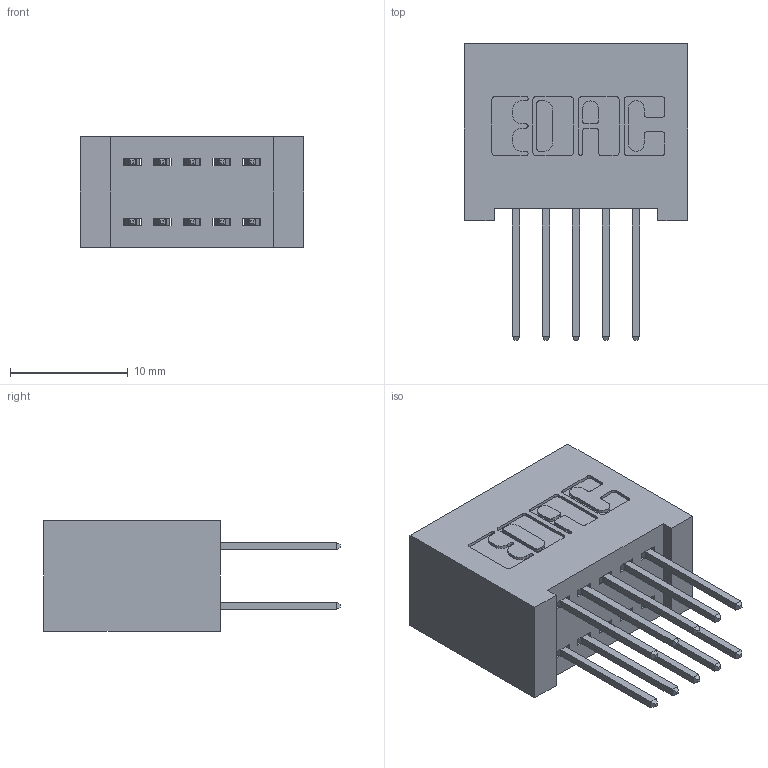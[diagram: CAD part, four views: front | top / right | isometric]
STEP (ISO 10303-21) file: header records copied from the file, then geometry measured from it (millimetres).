
FILE_DESCRIPTION (( 'STEP AP203' ), '1' );
FILE_NAME ('392-010-523-201.STEP', '2019-10-05T00:40:44', ( '' ), ( '' ), 'SwSTEP 2.0', 'SolidWorks 2016', '' );
FILE_SCHEMA (( 'CONFIG_CONTROL_DESIGN' ));
Length unit declared in the file: inch
Products named in the file (3): 392-010-523-201; 345-292-001_345-293-123; 342 Part_Lugless
Assembly tree (11 placements, depth 2):
  392-010-523-201
    342 Part_Lugless
    345-292-001_345-293-123  x10
Bounding box: 18.95 x 25.15 x 9.4 mm (x, y, z)
Volume: 1987.4 mm3; surface area: 2856.7 mm2
Topology: 11 solids, 11 shells, 622 faces, 1825 edges, 1202 vertices
Faces by surface type: plane 422, cylinder 200
Entity records: 7611 total; most frequent: CARTESIAN_POINT 1302, ORIENTED_EDGE 1238, DIRECTION 1171, EDGE_CURVE 619, LINE 499, VECTOR 499, VERTEX_POINT 410, AXIS2_PLACEMENT_3D 336
